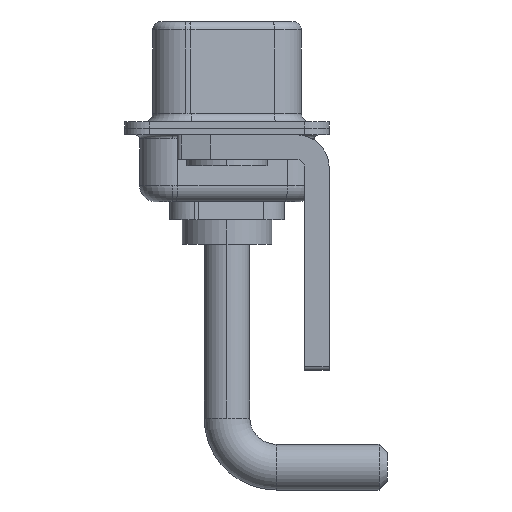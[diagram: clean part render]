
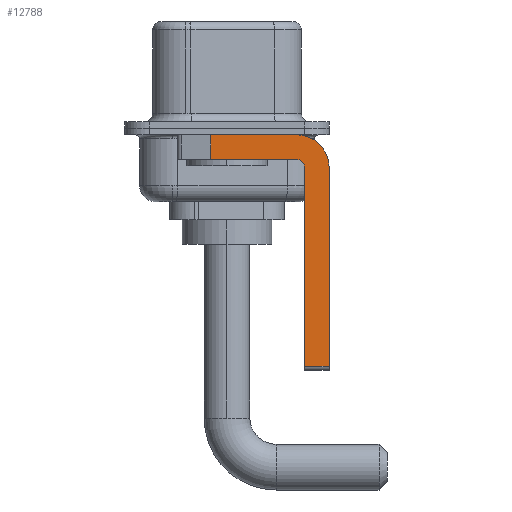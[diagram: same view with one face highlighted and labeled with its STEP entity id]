
A CAD part, left-side view. The second image highlights one B-rep face of the part: STEP entity #12788.
In plain terms, the highlighted planar face has unit normal (-1, 0, 0).
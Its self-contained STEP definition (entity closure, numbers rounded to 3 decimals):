
#221 = AXIS2_PLACEMENT_3D ( 'NONE', #10783, #8308, #13370 ) ;
#406 = AXIS2_PLACEMENT_3D ( 'NONE', #6153, #6235, #11671 ) ;
#667 = FACE_OUTER_BOUND ( 'NONE', #12452, .T. ) ;
#726 = CARTESIAN_POINT ( 'NONE',  ( -2.9, 0.978, -1.9 ) ) ;
#1484 = EDGE_CURVE ( 'NONE', #14371, #15011, #15919, .T. ) ;
#1606 = VECTOR ( 'NONE', #11642, 1000. ) ;
#1694 = DIRECTION ( 'NONE',  ( 0., 0., -1. ) ) ;
#2022 = DIRECTION ( 'NONE',  ( 0., -1., 0. ) ) ;
#2064 = VECTOR ( 'NONE', #11907, 1000. ) ;
#2126 = EDGE_CURVE ( 'NONE', #11354, #15801, #6711, .T. ) ;
#2344 = AXIS2_PLACEMENT_3D ( 'NONE', #11429, #16663, #4981 ) ;
#2356 = ORIENTED_EDGE ( 'NONE', *, *, #2126, .T. ) ;
#2363 = ORIENTED_EDGE ( 'NONE', *, *, #5371, .T. ) ;
#2388 = CARTESIAN_POINT ( 'NONE',  ( -2.9, 0.978, -1.9 ) ) ;
#2707 = VERTEX_POINT ( 'NONE', #15683 ) ;
#2721 = CARTESIAN_POINT ( 'NONE',  ( -2.9, -6.25, -14.55 ) ) ;
#2814 = CARTESIAN_POINT ( 'NONE',  ( -2.9, -4.25, -14.55 ) ) ;
#2938 = CARTESIAN_POINT ( 'NONE',  ( -2.9, -4.25, -1.9 ) ) ;
#2989 = VECTOR ( 'NONE', #4588, 1000. ) ;
#3578 = CARTESIAN_POINT ( 'NONE',  ( -2.9, -4.75, -2.4 ) ) ;
#3991 = EDGE_CURVE ( 'NONE', #15143, #15741, #4254, .T. ) ;
#4091 = LINE ( 'NONE', #14635, #8704 ) ;
#4254 = CIRCLE ( 'NONE', #2344, 2. ) ;
#4588 = DIRECTION ( 'NONE',  ( 0., 0., 1. ) ) ;
#4981 = DIRECTION ( 'NONE',  ( 0., 0., -1. ) ) ;
#5039 = CARTESIAN_POINT ( 'NONE',  ( -2.9, -4.75, -14.55 ) ) ;
#5371 = EDGE_CURVE ( 'NONE', #2707, #16605, #12929, .T. ) ;
#5558 = ORIENTED_EDGE ( 'NONE', *, *, #15976, .F. ) ;
#5621 = VECTOR ( 'NONE', #6177, 1000. ) ;
#5677 = EDGE_CURVE ( 'NONE', #11354, #14371, #5947, .T. ) ;
#5940 = LINE ( 'NONE', #14797, #15159 ) ;
#5947 = LINE ( 'NONE', #12229, #2989 ) ;
#6153 = CARTESIAN_POINT ( 'NONE',  ( -2.9, -4.25, -2.4 ) ) ;
#6177 = DIRECTION ( 'NONE',  ( 0., 1., 0. ) ) ;
#6235 = DIRECTION ( 'NONE',  ( -1., 0., 0. ) ) ;
#6711 = LINE ( 'NONE', #2814, #2064 ) ;
#7972 = EDGE_CURVE ( 'NONE', #15011, #16605, #13353, .T. ) ;
#8308 = DIRECTION ( 'NONE',  ( 1., 0., 0. ) ) ;
#8550 = ORIENTED_EDGE ( 'NONE', *, *, #1484, .F. ) ;
#8704 = VECTOR ( 'NONE', #1694, 1000. ) ;
#9582 = ORIENTED_EDGE ( 'NONE', *, *, #3991, .F. ) ;
#10473 = EDGE_CURVE ( 'NONE', #2707, #15143, #5940, .T. ) ;
#10783 = CARTESIAN_POINT ( 'NONE',  ( -2.9, -4.25, -2.4 ) ) ;
#11354 = VERTEX_POINT ( 'NONE', #5039 ) ;
#11429 = CARTESIAN_POINT ( 'NONE',  ( -2.9, -4.25, -2.4 ) ) ;
#11642 = DIRECTION ( 'NONE',  ( 0., 0., -1. ) ) ;
#11671 = DIRECTION ( 'NONE',  ( 0., 0., 1. ) ) ;
#11907 = DIRECTION ( 'NONE',  ( 0., -1., 0. ) ) ;
#12047 = CARTESIAN_POINT ( 'NONE',  ( -2.9, -4.25, -1.9 ) ) ;
#12229 = CARTESIAN_POINT ( 'NONE',  ( -2.9, -4.75, -14.8 ) ) ;
#12452 = EDGE_LOOP ( 'NONE', ( #13133, #2363, #14098, #8550, #12512, #2356, #5558, #9582 ) ) ;
#12512 = ORIENTED_EDGE ( 'NONE', *, *, #5677, .F. ) ;
#12788 = ADVANCED_FACE ( 'NONE', ( #667 ), #14726, .F. ) ;
#12929 = LINE ( 'NONE', #2388, #1606 ) ;
#13133 = ORIENTED_EDGE ( 'NONE', *, *, #10473, .F. ) ;
#13353 = LINE ( 'NONE', #12047, #5621 ) ;
#13370 = DIRECTION ( 'NONE',  ( 0., 0., -1. ) ) ;
#13964 = CARTESIAN_POINT ( 'NONE',  ( -2.9, -6.25, -2.4 ) ) ;
#14098 = ORIENTED_EDGE ( 'NONE', *, *, #7972, .F. ) ;
#14371 = VERTEX_POINT ( 'NONE', #3578 ) ;
#14635 = CARTESIAN_POINT ( 'NONE',  ( -2.9, -6.25, -2.4 ) ) ;
#14726 = PLANE ( 'NONE',  #221 ) ;
#14797 = CARTESIAN_POINT ( 'NONE',  ( -2.9, 3., -0.4 ) ) ;
#15011 = VERTEX_POINT ( 'NONE', #2938 ) ;
#15111 = CARTESIAN_POINT ( 'NONE',  ( -2.9, -4.25, -0.4 ) ) ;
#15143 = VERTEX_POINT ( 'NONE', #15111 ) ;
#15159 = VECTOR ( 'NONE', #2022, 1000. ) ;
#15683 = CARTESIAN_POINT ( 'NONE',  ( -2.9, 0.978, -0.4 ) ) ;
#15741 = VERTEX_POINT ( 'NONE', #13964 ) ;
#15801 = VERTEX_POINT ( 'NONE', #2721 ) ;
#15919 = CIRCLE ( 'NONE', #406, 0.5 ) ;
#15976 = EDGE_CURVE ( 'NONE', #15741, #15801, #4091, .T. ) ;
#16605 = VERTEX_POINT ( 'NONE', #726 ) ;
#16663 = DIRECTION ( 'NONE',  ( 1., 0., 0. ) ) ;
